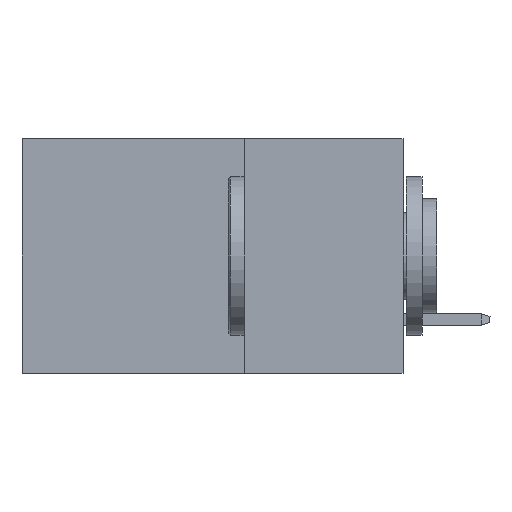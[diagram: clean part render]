
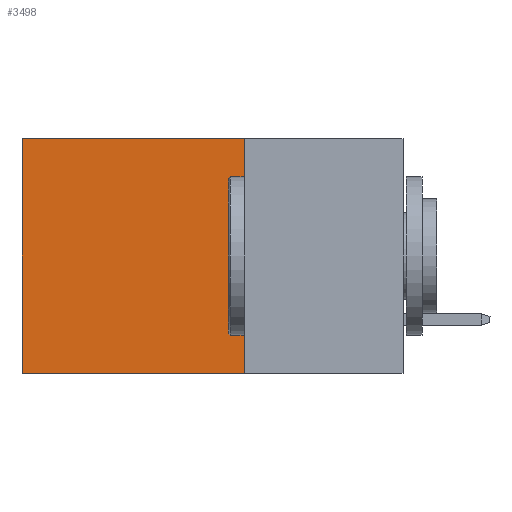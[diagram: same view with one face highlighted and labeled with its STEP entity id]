
A CAD part, left-side view. The second image highlights one B-rep face of the part: STEP entity #3498.
In plain terms, the highlighted planar face has unit normal (-1, 0, 0).
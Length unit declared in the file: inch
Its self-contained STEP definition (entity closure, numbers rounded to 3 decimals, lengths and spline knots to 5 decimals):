
#82 = LINE ( 'NONE', #4325, #2374 ) ;
#116 = CARTESIAN_POINT ( 'NONE',  ( 0.2875, 0.25, 0. ) ) ;
#139 = CARTESIAN_POINT ( 'NONE',  ( 0.2875, 0.25, 0. ) ) ;
#426 = CARTESIAN_POINT ( 'NONE',  ( 0.2875, 0.6, 0. ) ) ;
#772 = ORIENTED_EDGE ( 'NONE', *, *, #1059, .T. ) ;
#1059 = EDGE_CURVE ( 'NONE', #8855, #3463, #3763, .T. ) ;
#1096 = ORIENTED_EDGE ( 'NONE', *, *, #3803, .T. ) ;
#1103 = DIRECTION ( 'NONE',  ( 0., 0., -1. ) ) ;
#1272 = CARTESIAN_POINT ( 'NONE',  ( 0.2875, 0.25, -0.37 ) ) ;
#1478 = CARTESIAN_POINT ( 'NONE',  ( 0.2875, 0.25, -0.37 ) ) ;
#1943 = ORIENTED_EDGE ( 'NONE', *, *, #9549, .F. ) ;
#2047 = DIRECTION ( 'NONE',  ( 1., 0., 0. ) ) ;
#2144 = VERTEX_POINT ( 'NONE', #1272 ) ;
#2266 = FACE_OUTER_BOUND ( 'NONE', #9123, .T. ) ;
#2374 = VECTOR ( 'NONE', #5957, 39.37008 ) ;
#2889 = AXIS2_PLACEMENT_3D ( 'NONE', #7048, #2047, #10386 ) ;
#3463 = VERTEX_POINT ( 'NONE', #426 ) ;
#3498 = ADVANCED_FACE ( 'NONE', ( #2266 ), #7099, .F. ) ;
#3739 = VERTEX_POINT ( 'NONE', #7462 ) ;
#3763 = LINE ( 'NONE', #10365, #4947 ) ;
#3803 = EDGE_CURVE ( 'NONE', #3463, #3739, #82, .T. ) ;
#4084 = LINE ( 'NONE', #1478, #9877 ) ;
#4233 = EDGE_CURVE ( 'NONE', #8855, #2144, #4417, .T. ) ;
#4325 = CARTESIAN_POINT ( 'NONE',  ( 0.2875, 0.6, 0. ) ) ;
#4417 = LINE ( 'NONE', #116, #5854 ) ;
#4423 = ORIENTED_EDGE ( 'NONE', *, *, #4233, .F. ) ;
#4947 = VECTOR ( 'NONE', #9548, 39.37008 ) ;
#5721 = DIRECTION ( 'NONE',  ( 0., 1., 0. ) ) ;
#5854 = VECTOR ( 'NONE', #1103, 39.37008 ) ;
#5957 = DIRECTION ( 'NONE',  ( 0., 0., -1. ) ) ;
#7048 = CARTESIAN_POINT ( 'NONE',  ( 0.2875, 0.25, 0. ) ) ;
#7099 = PLANE ( 'NONE',  #2889 ) ;
#7462 = CARTESIAN_POINT ( 'NONE',  ( 0.2875, 0.6, -0.37 ) ) ;
#8855 = VERTEX_POINT ( 'NONE', #139 ) ;
#9123 = EDGE_LOOP ( 'NONE', ( #1096, #1943, #4423, #772 ) ) ;
#9548 = DIRECTION ( 'NONE',  ( 0., 1., 0. ) ) ;
#9549 = EDGE_CURVE ( 'NONE', #2144, #3739, #4084, .T. ) ;
#9877 = VECTOR ( 'NONE', #5721, 39.37008 ) ;
#10365 = CARTESIAN_POINT ( 'NONE',  ( 0.2875, 0.25, 0. ) ) ;
#10386 = DIRECTION ( 'NONE',  ( 0., 0., -1. ) ) ;
